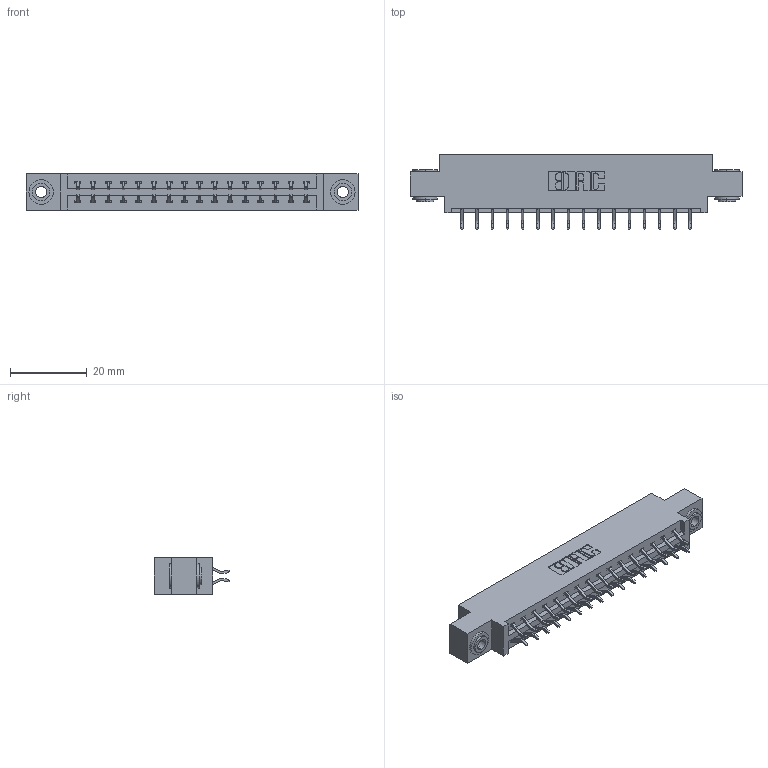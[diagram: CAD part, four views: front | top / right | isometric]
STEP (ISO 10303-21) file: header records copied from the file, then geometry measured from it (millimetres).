
FILE_DESCRIPTION (( 'STEP AP203' ), '1' );
FILE_NAME ('387-032-556-803.STEP', '2019-10-17T16:24:38', ( '' ), ( '' ), 'SwSTEP 2.0', 'SolidWorks 2016', '' );
FILE_SCHEMA (( 'CONFIG_CONTROL_DESIGN' ));
Length unit declared in the file: inch
Products named in the file (4): 337 Part_0.170 Offset - 0.156 Dia-TH; 345-292-001_556 Tail; 345-250-002_345-250-002-102; 387-032-556-803
Assembly tree (35 placements, depth 2):
  387-032-556-803
    337 Part_0.170 Offset - 0.156 Dia-TH
    345-292-001_556 Tail  x32
    345-250-002_345-250-002-102  x2
Bounding box: 86.41 x 19.57 x 9.4 mm (x, y, z)
Volume: 8661.2 mm3; surface area: 9837.4 mm2
Topology: 35 solids, 35 shells, 2076 faces, 6127 edges, 4038 vertices
Faces by surface type: plane 1428, cylinder 640, cone 8
Entity records: 16770 total; most frequent: CARTESIAN_POINT 2837, ORIENTED_EDGE 2754, DIRECTION 2483, EDGE_CURVE 1377, VECTOR 1217, LINE 1217, VERTEX_POINT 914, AXIS2_PLACEMENT_3D 633
